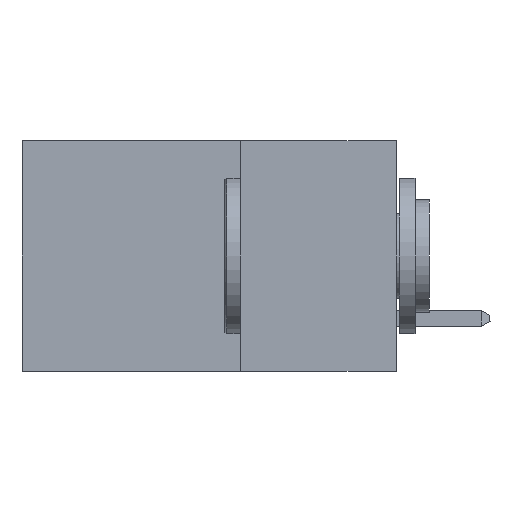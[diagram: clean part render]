
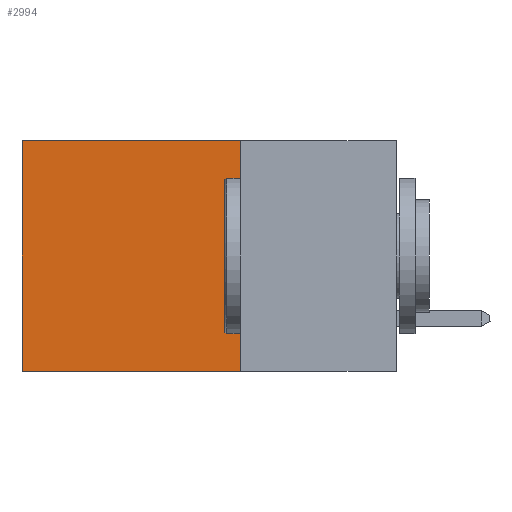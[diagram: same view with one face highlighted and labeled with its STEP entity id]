
A CAD part, left-side view. The second image highlights one B-rep face of the part: STEP entity #2994.
In plain terms, the highlighted planar face has unit normal (-1, 0, 0).
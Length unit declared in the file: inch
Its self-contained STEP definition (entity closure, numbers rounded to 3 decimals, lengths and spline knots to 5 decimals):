
#346 = VECTOR ( 'NONE', #13464, 39.37008 ) ;
#898 = ORIENTED_EDGE ( 'NONE', *, *, #8997, .F. ) ;
#2994 = ADVANCED_FACE ( 'NONE', ( #7044 ), #15920, .F. ) ;
#3633 = EDGE_CURVE ( 'NONE', #14776, #6934, #10213, .T. ) ;
#3794 = VECTOR ( 'NONE', #5975, 39.37008 ) ;
#3986 = DIRECTION ( 'NONE',  ( 0., 0., -1. ) ) ;
#4100 = CARTESIAN_POINT ( 'NONE',  ( 0.298, 0.25, 0. ) ) ;
#4144 = DIRECTION ( 'NONE',  ( 1., 0., 0. ) ) ;
#4341 = ORIENTED_EDGE ( 'NONE', *, *, #11809, .T. ) ;
#5010 = LINE ( 'NONE', #4100, #14793 ) ;
#5067 = CARTESIAN_POINT ( 'NONE',  ( 0.298, 0.6, 0. ) ) ;
#5139 = ORIENTED_EDGE ( 'NONE', *, *, #10792, .T. ) ;
#5429 = DIRECTION ( 'NONE',  ( 0., 1., 0. ) ) ;
#5785 = ORIENTED_EDGE ( 'NONE', *, *, #3633, .F. ) ;
#5975 = DIRECTION ( 'NONE',  ( 0., 0., -1. ) ) ;
#6031 = CARTESIAN_POINT ( 'NONE',  ( 0.298, 0.25, 0. ) ) ;
#6266 = VERTEX_POINT ( 'NONE', #5067 ) ;
#6461 = EDGE_LOOP ( 'NONE', ( #5139, #5785, #898, #4341 ) ) ;
#6816 = VECTOR ( 'NONE', #5429, 39.37008 ) ;
#6934 = VERTEX_POINT ( 'NONE', #15677 ) ;
#7044 = FACE_OUTER_BOUND ( 'NONE', #6461, .T. ) ;
#7140 = CARTESIAN_POINT ( 'NONE',  ( 0.298, 0.6, 0. ) ) ;
#7573 = LINE ( 'NONE', #7140, #346 ) ;
#7885 = CARTESIAN_POINT ( 'NONE',  ( 0.298, 0.25, 0. ) ) ;
#8997 = EDGE_CURVE ( 'NONE', #15736, #14776, #14002, .T. ) ;
#10140 = AXIS2_PLACEMENT_3D ( 'NONE', #14311, #4144, #3986 ) ;
#10213 = LINE ( 'NONE', #11849, #6816 ) ;
#10542 = DIRECTION ( 'NONE',  ( 0., 1., 0. ) ) ;
#10792 = EDGE_CURVE ( 'NONE', #6266, #6934, #7573, .T. ) ;
#11809 = EDGE_CURVE ( 'NONE', #15736, #6266, #5010, .T. ) ;
#11849 = CARTESIAN_POINT ( 'NONE',  ( 0.298, 0.25, -0.37 ) ) ;
#12402 = CARTESIAN_POINT ( 'NONE',  ( 0.298, 0.25, -0.37 ) ) ;
#13464 = DIRECTION ( 'NONE',  ( 0., 0., -1. ) ) ;
#14002 = LINE ( 'NONE', #6031, #3794 ) ;
#14311 = CARTESIAN_POINT ( 'NONE',  ( 0.298, 0.25, 0. ) ) ;
#14776 = VERTEX_POINT ( 'NONE', #12402 ) ;
#14793 = VECTOR ( 'NONE', #10542, 39.37008 ) ;
#15677 = CARTESIAN_POINT ( 'NONE',  ( 0.298, 0.6, -0.37 ) ) ;
#15736 = VERTEX_POINT ( 'NONE', #7885 ) ;
#15920 = PLANE ( 'NONE',  #10140 ) ;
